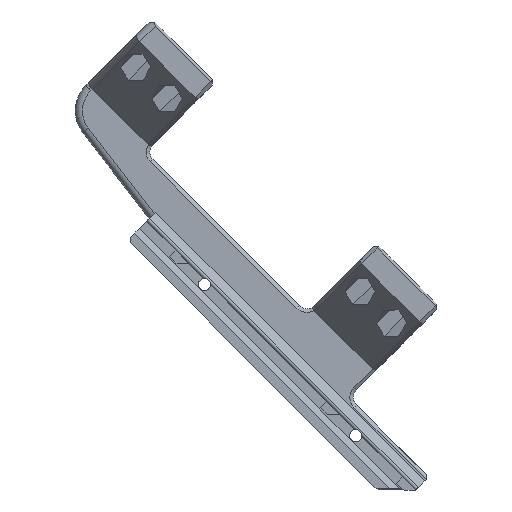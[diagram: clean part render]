
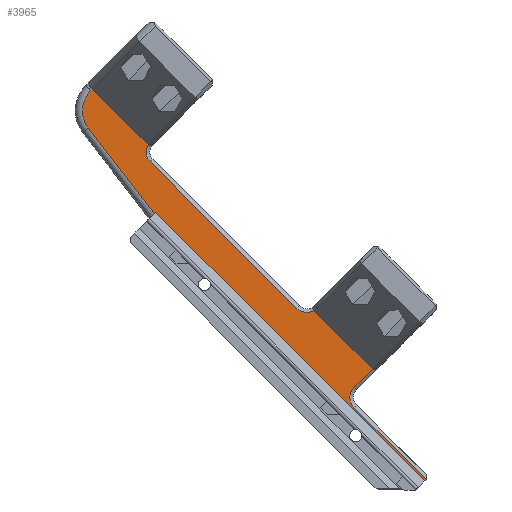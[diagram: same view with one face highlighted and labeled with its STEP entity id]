
A CAD part, left-side view. The second image highlights one B-rep face of the part: STEP entity #3965.
In plain terms, the highlighted planar face has unit normal (-1, 0, 0).
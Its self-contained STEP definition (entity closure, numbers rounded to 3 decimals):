
#154=CIRCLE('',#4223,8.);
#156=CIRCLE('',#4229,4.);
#157=CIRCLE('',#4230,4.);
#158=CIRCLE('',#4231,4.);
#226=FACE_OUTER_BOUND('',#446,.T.);
#446=EDGE_LOOP('',(#2757,#2758,#2759,#2760,#2761,#2762,#2763,#2764,#2765,
#2766,#2767,#2768,#2769,#2770));
#716=LINE('',#5693,#1167);
#726=LINE('',#5723,#1177);
#752=LINE('',#5781,#1203);
#753=LINE('',#5793,#1204);
#756=LINE('',#5799,#1207);
#757=LINE('',#5801,#1208);
#758=LINE('',#5805,#1209);
#759=LINE('',#5807,#1210);
#760=LINE('',#5811,#1211);
#761=LINE('',#5814,#1212);
#1167=VECTOR('',#4577,10.);
#1177=VECTOR('',#4591,10.);
#1203=VECTOR('',#4635,10.);
#1204=VECTOR('',#4652,10.);
#1207=VECTOR('',#4659,10.);
#1208=VECTOR('',#4660,10.);
#1209=VECTOR('',#4663,10.);
#1210=VECTOR('',#4664,10.);
#1211=VECTOR('',#4667,10.);
#1212=VECTOR('',#4670,10.);
#1669=VERTEX_POINT('',#5690);
#1670=VERTEX_POINT('',#5692);
#1680=VERTEX_POINT('',#5721);
#1702=VERTEX_POINT('',#5779);
#1703=VERTEX_POINT('',#5780);
#1704=VERTEX_POINT('',#5785);
#1707=VERTEX_POINT('',#5798);
#1708=VERTEX_POINT('',#5800);
#1709=VERTEX_POINT('',#5802);
#1710=VERTEX_POINT('',#5804);
#1711=VERTEX_POINT('',#5806);
#1712=VERTEX_POINT('',#5808);
#1713=VERTEX_POINT('',#5810);
#1714=VERTEX_POINT('',#5812);
#2069=EDGE_CURVE('',#1670,#1669,#716,.T.);
#2081=EDGE_CURVE('',#1680,#1669,#726,.F.);
#2109=EDGE_CURVE('',#1702,#1703,#752,.T.);
#2113=EDGE_CURVE('',#1703,#1704,#154,.T.);
#2116=EDGE_CURVE('',#1704,#1670,#753,.T.);
#2119=EDGE_CURVE('',#1680,#1707,#756,.T.);
#2120=EDGE_CURVE('',#1707,#1708,#757,.T.);
#2121=EDGE_CURVE('',#1708,#1709,#156,.T.);
#2122=EDGE_CURVE('',#1709,#1710,#758,.T.);
#2123=EDGE_CURVE('',#1711,#1710,#759,.T.);
#2124=EDGE_CURVE('',#1711,#1712,#157,.T.);
#2125=EDGE_CURVE('',#1712,#1713,#760,.T.);
#2126=EDGE_CURVE('',#1713,#1714,#158,.T.);
#2127=EDGE_CURVE('',#1702,#1714,#761,.T.);
#2757=ORIENTED_EDGE('',*,*,#2116,.T.);
#2758=ORIENTED_EDGE('',*,*,#2069,.T.);
#2759=ORIENTED_EDGE('',*,*,#2081,.F.);
#2760=ORIENTED_EDGE('',*,*,#2119,.T.);
#2761=ORIENTED_EDGE('',*,*,#2120,.T.);
#2762=ORIENTED_EDGE('',*,*,#2121,.T.);
#2763=ORIENTED_EDGE('',*,*,#2122,.T.);
#2764=ORIENTED_EDGE('',*,*,#2123,.F.);
#2765=ORIENTED_EDGE('',*,*,#2124,.T.);
#2766=ORIENTED_EDGE('',*,*,#2125,.T.);
#2767=ORIENTED_EDGE('',*,*,#2126,.T.);
#2768=ORIENTED_EDGE('',*,*,#2127,.F.);
#2769=ORIENTED_EDGE('',*,*,#2109,.T.);
#2770=ORIENTED_EDGE('',*,*,#2113,.T.);
#3793=PLANE('',#4228);
#3965=ADVANCED_FACE('',(#226),#3793,.F.);
#4223=AXIS2_PLACEMENT_3D('',#5788,#4644,#4645);
#4228=AXIS2_PLACEMENT_3D('',#5797,#4657,#4658);
#4229=AXIS2_PLACEMENT_3D('',#5803,#4661,#4662);
#4230=AXIS2_PLACEMENT_3D('',#5809,#4665,#4666);
#4231=AXIS2_PLACEMENT_3D('',#5813,#4668,#4669);
#4577=DIRECTION('',(0.,-0.707,0.707));
#4591=DIRECTION('',(0.,-0.707,-0.707));
#4635=DIRECTION('',(0.,0.707,-0.707));
#4644=DIRECTION('center_axis',(-1.,0.,0.));
#4645=DIRECTION('ref_axis',(0.,0.998,0.064));
#4652=DIRECTION('',(0.,-0.611,-0.791));
#4657=DIRECTION('center_axis',(1.,0.,0.));
#4658=DIRECTION('ref_axis',(0.,0.707,0.707));
#4659=DIRECTION('',(0.,-0.707,0.707));
#4660=DIRECTION('',(0.,0.707,0.707));
#4661=DIRECTION('center_axis',(1.,0.,0.));
#4662=DIRECTION('ref_axis',(0.,1.,0.));
#4663=DIRECTION('',(0.,-0.707,0.707));
#4664=DIRECTION('',(0.,-0.707,-0.707));
#4665=DIRECTION('center_axis',(1.,0.,0.));
#4666=DIRECTION('ref_axis',(0.,0.,-1.));
#4667=DIRECTION('',(0.,0.707,0.707));
#4668=DIRECTION('center_axis',(1.,0.,0.));
#4669=DIRECTION('ref_axis',(0.,1.,0.));
#4670=DIRECTION('',(0.,-0.707,-0.707));
#5690=CARTESIAN_POINT('',(-8.23,90.288,80.498));
#5692=CARTESIAN_POINT('',(-8.23,90.707,80.078));
#5693=CARTESIAN_POINT('',(-8.23,91.425,79.361));
#5721=CARTESIAN_POINT('',(-8.23,14.91,5.12));
#5723=CARTESIAN_POINT('',(-8.23,24.173,14.384));
#5779=CARTESIAN_POINT('',(-8.23,108.123,114.988));
#5780=CARTESIAN_POINT('',(-8.23,108.538,114.574));
#5781=CARTESIAN_POINT('',(-8.23,115.336,107.775));
#5785=CARTESIAN_POINT('',(-8.23,109.211,104.025));
#5788=CARTESIAN_POINT('Origin',(-8.23,102.881,108.917));
#5793=CARTESIAN_POINT('',(-8.23,73.982,58.433));
#5797=CARTESIAN_POINT('Origin',(-8.23,36.14,28.579));
#5798=CARTESIAN_POINT('',(-8.23,14.503,5.528));
#5799=CARTESIAN_POINT('',(-8.23,10.146,9.885));
#5800=CARTESIAN_POINT('',(-8.23,34.726,25.751));
#5801=CARTESIAN_POINT('',(-8.23,23.766,14.791));
#5802=CARTESIAN_POINT('',(-8.23,34.726,31.408));
#5803=CARTESIAN_POINT('Origin',(-8.23,31.898,28.579));
#5804=CARTESIAN_POINT('',(-8.23,29.634,36.5));
#5805=CARTESIAN_POINT('',(-8.23,36.848,29.286));
#5806=CARTESIAN_POINT('',(-8.23,46.01,52.875));
#5807=CARTESIAN_POINT('',(-8.23,28.927,35.792));
#5808=CARTESIAN_POINT('',(-8.23,50.767,53.551));
#5809=CARTESIAN_POINT('Origin',(-8.23,47.939,56.379));
#5810=CARTESIAN_POINT('',(-8.23,91.779,94.563));
#5811=CARTESIAN_POINT('',(-8.23,51.121,53.904));
#5812=CARTESIAN_POINT('',(-8.23,92.455,99.32));
#5813=CARTESIAN_POINT('Origin',(-8.23,88.951,97.391));
#5814=CARTESIAN_POINT('',(-8.23,60.394,67.259));
